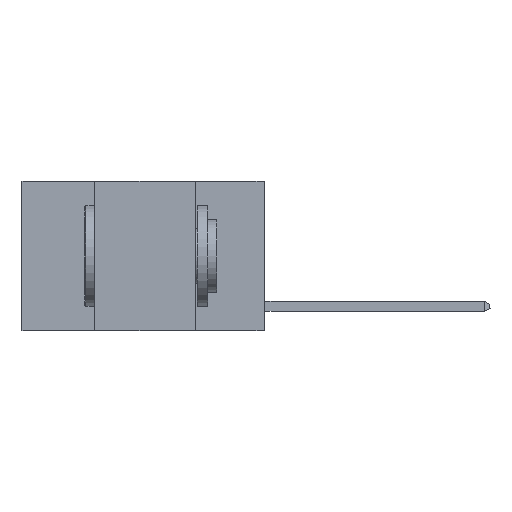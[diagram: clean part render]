
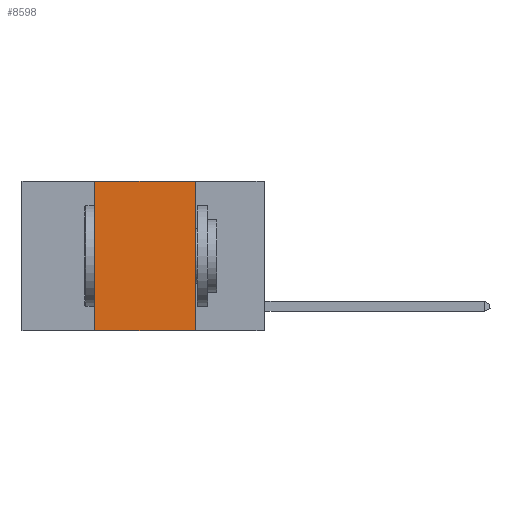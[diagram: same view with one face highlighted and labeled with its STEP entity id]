
A CAD part, left-side view. The second image highlights one B-rep face of the part: STEP entity #8598.
In plain terms, the highlighted planar face has unit normal (-1, 0, 0).
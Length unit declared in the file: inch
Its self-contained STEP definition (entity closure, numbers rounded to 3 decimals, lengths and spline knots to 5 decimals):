
#714 = CARTESIAN_POINT ( 'NONE',  ( 0., 0.6, 0. ) ) ;
#1305 = VERTEX_POINT ( 'NONE', #5649 ) ;
#2254 = VECTOR ( 'NONE', #17546, 39.37008 ) ;
#4185 = VERTEX_POINT ( 'NONE', #18173 ) ;
#4871 = ORIENTED_EDGE ( 'NONE', *, *, #24683, .F. ) ;
#5120 = LINE ( 'NONE', #714, #20121 ) ;
#5263 = ORIENTED_EDGE ( 'NONE', *, *, #23719, .F. ) ;
#5486 = DIRECTION ( 'NONE',  ( 0., 0., -1. ) ) ;
#5649 = CARTESIAN_POINT ( 'NONE',  ( 0., 0.17, 0. ) ) ;
#5827 = LINE ( 'NONE', #23805, #2254 ) ;
#6434 = EDGE_CURVE ( 'NONE', #17249, #4185, #23859, .T. ) ;
#6513 = DIRECTION ( 'NONE',  ( 0., 0., -1. ) ) ;
#7655 = ORIENTED_EDGE ( 'NONE', *, *, #6434, .T. ) ;
#8225 = CARTESIAN_POINT ( 'NONE',  ( 0., 0.6, 0. ) ) ;
#8567 = DIRECTION ( 'NONE',  ( 0., -1., 0. ) ) ;
#8598 = ADVANCED_FACE ( 'NONE', ( #23742 ), #22481, .F. ) ;
#8733 = VECTOR ( 'NONE', #19978, 39.37008 ) ;
#9723 = CARTESIAN_POINT ( 'NONE',  ( 0., 0.6, -0.37 ) ) ;
#10079 = EDGE_LOOP ( 'NONE', ( #16984, #5263, #4871, #7655 ) ) ;
#12600 = CARTESIAN_POINT ( 'NONE',  ( 0., 0.42, 0. ) ) ;
#15774 = VECTOR ( 'NONE', #6513, 39.37008 ) ;
#15776 = CARTESIAN_POINT ( 'NONE',  ( 0., 0.42, -0.37 ) ) ;
#16984 = ORIENTED_EDGE ( 'NONE', *, *, #19489, .F. ) ;
#17249 = VERTEX_POINT ( 'NONE', #15776 ) ;
#17546 = DIRECTION ( 'NONE',  ( 0., 0., 1. ) ) ;
#18173 = CARTESIAN_POINT ( 'NONE',  ( 0., 0.17, -0.37 ) ) ;
#18295 = VERTEX_POINT ( 'NONE', #12600 ) ;
#19489 = EDGE_CURVE ( 'NONE', #1305, #4185, #24759, .T. ) ;
#19730 = DIRECTION ( 'NONE',  ( 1., 0., 0. ) ) ;
#19978 = DIRECTION ( 'NONE',  ( 0., -1., 0. ) ) ;
#20121 = VECTOR ( 'NONE', #8567, 39.37008 ) ;
#22481 = PLANE ( 'NONE',  #25868 ) ;
#23719 = EDGE_CURVE ( 'NONE', #18295, #1305, #5120, .T. ) ;
#23742 = FACE_OUTER_BOUND ( 'NONE', #10079, .T. ) ;
#23805 = CARTESIAN_POINT ( 'NONE',  ( 0., 0.42, 0. ) ) ;
#23859 = LINE ( 'NONE', #9723, #8733 ) ;
#24683 = EDGE_CURVE ( 'NONE', #17249, #18295, #5827, .T. ) ;
#24759 = LINE ( 'NONE', #24887, #15774 ) ;
#24887 = CARTESIAN_POINT ( 'NONE',  ( 0., 0.17, 0. ) ) ;
#25868 = AXIS2_PLACEMENT_3D ( 'NONE', #8225, #19730, #5486 ) ;
